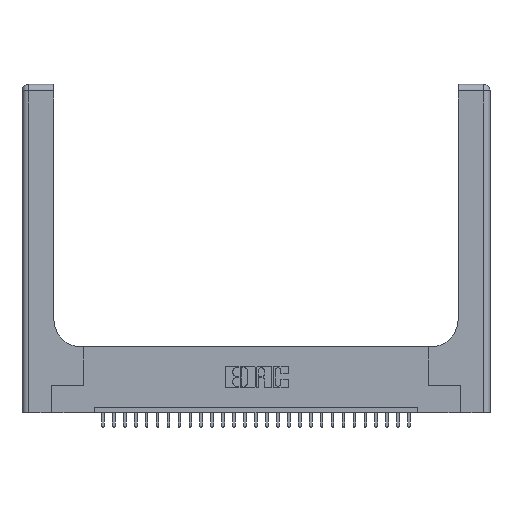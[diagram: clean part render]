
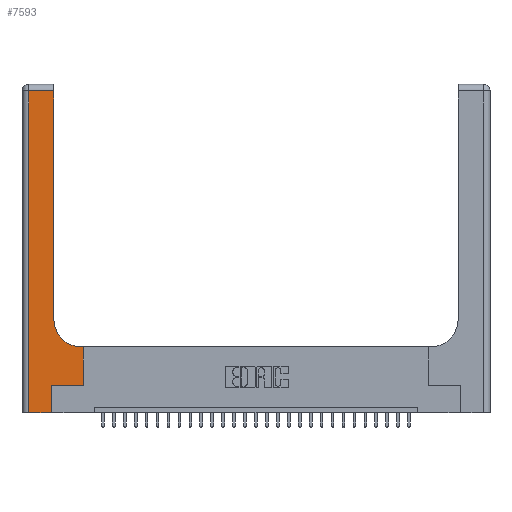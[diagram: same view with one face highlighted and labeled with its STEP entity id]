
A CAD part, top view. The second image highlights one B-rep face of the part: STEP entity #7593.
In plain terms, the highlighted planar face has unit normal (0, 0, 1).
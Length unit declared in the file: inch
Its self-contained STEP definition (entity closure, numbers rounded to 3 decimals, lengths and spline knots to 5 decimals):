
#128 = DIRECTION ( 'NONE',  ( -1., 0., 0. ) ) ;
#177 = VERTEX_POINT ( 'NONE', #28287 ) ;
#307 = VECTOR ( 'NONE', #128, 39.37008 ) ;
#641 = LINE ( 'NONE', #20492, #8625 ) ;
#845 = LINE ( 'NONE', #25214, #13400 ) ;
#849 = ORIENTED_EDGE ( 'NONE', *, *, #3193, .T. ) ;
#1140 = CARTESIAN_POINT ( 'NONE',  ( 0.5415, 0.6, 0.37 ) ) ;
#1211 = LINE ( 'NONE', #5508, #18252 ) ;
#2125 = CARTESIAN_POINT ( 'NONE',  ( 0.5415, 0.85, 0.37 ) ) ;
#3193 = EDGE_CURVE ( 'NONE', #27600, #14325, #21068, .T. ) ;
#3796 = VECTOR ( 'NONE', #23938, 39.37008 ) ;
#3840 = CARTESIAN_POINT ( 'NONE',  ( 0.5585, 0.6, 0.37 ) ) ;
#3857 = ORIENTED_EDGE ( 'NONE', *, *, #14896, .T. ) ;
#3874 = VERTEX_POINT ( 'NONE', #26203 ) ;
#4395 = EDGE_CURVE ( 'NONE', #6917, #3874, #4964, .T. ) ;
#4766 = ORIENTED_EDGE ( 'NONE', *, *, #18977, .T. ) ;
#4825 = CARTESIAN_POINT ( 'NONE',  ( 0., 0., 0.37 ) ) ;
#4964 = CIRCLE ( 'NONE', #22163, 0.25 ) ;
#5221 = DIRECTION ( 'NONE',  ( 0., 1., 0. ) ) ;
#5508 = CARTESIAN_POINT ( 'NONE',  ( 0.269, 0., 0.37 ) ) ;
#6917 = VERTEX_POINT ( 'NONE', #1140 ) ;
#7077 = VERTEX_POINT ( 'NONE', #10736 ) ;
#7108 = AXIS2_PLACEMENT_3D ( 'NONE', #16098, #7306, #13969 ) ;
#7306 = DIRECTION ( 'NONE',  ( 0., 0., -1. ) ) ;
#7593 = ADVANCED_FACE ( 'NONE', ( #25294 ), #25016, .F. ) ;
#8615 = EDGE_LOOP ( 'NONE', ( #4766, #849, #25200, #3857, #11381, #13273, #11435, #27599, #24362 ) ) ;
#8625 = VECTOR ( 'NONE', #17623, 39.37008 ) ;
#9241 = CARTESIAN_POINT ( 'NONE',  ( 0., 2.94, 0.37 ) ) ;
#9673 = VECTOR ( 'NONE', #20296, 39.37008 ) ;
#10655 = VECTOR ( 'NONE', #20652, 39.37008 ) ;
#10736 = CARTESIAN_POINT ( 'NONE',  ( 0.06, 0., 0.37 ) ) ;
#11381 = ORIENTED_EDGE ( 'NONE', *, *, #15944, .T. ) ;
#11435 = ORIENTED_EDGE ( 'NONE', *, *, #24043, .T. ) ;
#11523 = DIRECTION ( 'NONE',  ( -1., 0., 0. ) ) ;
#11586 = EDGE_CURVE ( 'NONE', #15810, #6917, #23982, .T. ) ;
#12524 = LINE ( 'NONE', #21688, #3796 ) ;
#13082 = CARTESIAN_POINT ( 'NONE',  ( 0.269, 0., 0.37 ) ) ;
#13273 = ORIENTED_EDGE ( 'NONE', *, *, #19268, .T. ) ;
#13400 = VECTOR ( 'NONE', #27449, 39.37008 ) ;
#13848 = VERTEX_POINT ( 'NONE', #27677 ) ;
#13969 = DIRECTION ( 'NONE',  ( -1., 0., 0. ) ) ;
#14325 = VERTEX_POINT ( 'NONE', #26392 ) ;
#14896 = EDGE_CURVE ( 'NONE', #7077, #22854, #26660, .T. ) ;
#15199 = VECTOR ( 'NONE', #11523, 39.37008 ) ;
#15810 = VERTEX_POINT ( 'NONE', #3840 ) ;
#15944 = EDGE_CURVE ( 'NONE', #22854, #177, #1211, .T. ) ;
#16098 = CARTESIAN_POINT ( 'NONE',  ( 0., 3., 0.37 ) ) ;
#17623 = DIRECTION ( 'NONE',  ( 0., -1., 0. ) ) ;
#18252 = VECTOR ( 'NONE', #5221, 39.37008 ) ;
#18977 = EDGE_CURVE ( 'NONE', #3874, #27600, #25331, .T. ) ;
#19268 = EDGE_CURVE ( 'NONE', #177, #13848, #12524, .T. ) ;
#20296 = DIRECTION ( 'NONE',  ( 0., 1., 0. ) ) ;
#20492 = CARTESIAN_POINT ( 'NONE',  ( 0.06, 3., 0.37 ) ) ;
#20652 = DIRECTION ( 'NONE',  ( 1., 0., 0. ) ) ;
#21068 = LINE ( 'NONE', #9241, #15199 ) ;
#21642 = EDGE_CURVE ( 'NONE', #14325, #7077, #641, .T. ) ;
#21688 = CARTESIAN_POINT ( 'NONE',  ( 0.269, 0.25, 0.37 ) ) ;
#22045 = DIRECTION ( 'NONE',  ( 0., 0., -1. ) ) ;
#22163 = AXIS2_PLACEMENT_3D ( 'NONE', #2125, #22045, #24286 ) ;
#22854 = VERTEX_POINT ( 'NONE', #13082 ) ;
#23002 = CARTESIAN_POINT ( 'NONE',  ( 0.2915, 2.94, 0.37 ) ) ;
#23938 = DIRECTION ( 'NONE',  ( 1., 0., 0. ) ) ;
#23982 = LINE ( 'NONE', #24602, #307 ) ;
#24043 = EDGE_CURVE ( 'NONE', #13848, #15810, #845, .T. ) ;
#24286 = DIRECTION ( 'NONE',  ( 1., 0., 0. ) ) ;
#24362 = ORIENTED_EDGE ( 'NONE', *, *, #4395, .T. ) ;
#24602 = CARTESIAN_POINT ( 'NONE',  ( 0.2915, 0.6, 0.37 ) ) ;
#25016 = PLANE ( 'NONE',  #7108 ) ;
#25200 = ORIENTED_EDGE ( 'NONE', *, *, #21642, .T. ) ;
#25214 = CARTESIAN_POINT ( 'NONE',  ( 0.5585, 0.25, 0.37 ) ) ;
#25294 = FACE_OUTER_BOUND ( 'NONE', #8615, .T. ) ;
#25331 = LINE ( 'NONE', #26155, #9673 ) ;
#26155 = CARTESIAN_POINT ( 'NONE',  ( 0.2915, 3., 0.37 ) ) ;
#26203 = CARTESIAN_POINT ( 'NONE',  ( 0.2915, 0.85, 0.37 ) ) ;
#26392 = CARTESIAN_POINT ( 'NONE',  ( 0.06, 2.94, 0.37 ) ) ;
#26660 = LINE ( 'NONE', #4825, #10655 ) ;
#27449 = DIRECTION ( 'NONE',  ( 0., 1., 0. ) ) ;
#27599 = ORIENTED_EDGE ( 'NONE', *, *, #11586, .T. ) ;
#27600 = VERTEX_POINT ( 'NONE', #23002 ) ;
#27677 = CARTESIAN_POINT ( 'NONE',  ( 0.5585, 0.25, 0.37 ) ) ;
#28287 = CARTESIAN_POINT ( 'NONE',  ( 0.269, 0.25, 0.37 ) ) ;
